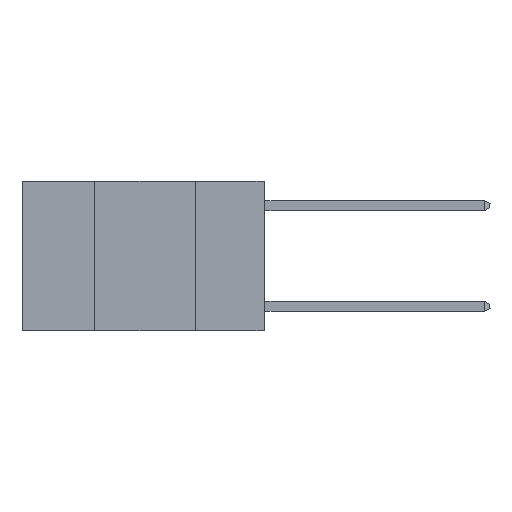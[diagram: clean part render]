
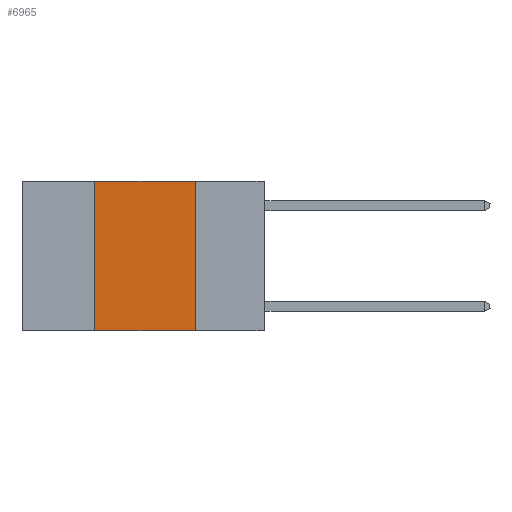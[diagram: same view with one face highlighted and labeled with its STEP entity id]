
A CAD part, left-side view. The second image highlights one B-rep face of the part: STEP entity #6965.
In plain terms, the highlighted planar face has unit normal (-1, 0, 0).
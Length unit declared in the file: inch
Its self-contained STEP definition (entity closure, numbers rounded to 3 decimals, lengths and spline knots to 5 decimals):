
#313 = EDGE_LOOP ( 'NONE', ( #2954, #5446, #2824, #8068 ) ) ;
#497 = CARTESIAN_POINT ( 'NONE',  ( 0., 0.6, 0. ) ) ;
#571 = EDGE_CURVE ( 'NONE', #6247, #1300, #6232, .T. ) ;
#786 = LINE ( 'NONE', #5192, #2354 ) ;
#1005 = CARTESIAN_POINT ( 'NONE',  ( 0., 0.17, -0.37 ) ) ;
#1020 = DIRECTION ( 'NONE',  ( 0., -1., 0. ) ) ;
#1263 = CARTESIAN_POINT ( 'NONE',  ( 0., 0.42, -0.37 ) ) ;
#1300 = VERTEX_POINT ( 'NONE', #2081 ) ;
#1341 = LINE ( 'NONE', #1488, #8252 ) ;
#1369 = VECTOR ( 'NONE', #8205, 39.37008 ) ;
#1441 = DIRECTION ( 'NONE',  ( 0., 0., 1. ) ) ;
#1488 = CARTESIAN_POINT ( 'NONE',  ( 0., 0.42, 0. ) ) ;
#1501 = DIRECTION ( 'NONE',  ( 0., 0., -1. ) ) ;
#2030 = FACE_OUTER_BOUND ( 'NONE', #313, .T. ) ;
#2081 = CARTESIAN_POINT ( 'NONE',  ( 0., 0.17, 0. ) ) ;
#2354 = VECTOR ( 'NONE', #1501, 39.37008 ) ;
#2787 = CARTESIAN_POINT ( 'NONE',  ( 0., 0.42, 0. ) ) ;
#2824 = ORIENTED_EDGE ( 'NONE', *, *, #7184, .F. ) ;
#2954 = ORIENTED_EDGE ( 'NONE', *, *, #6688, .F. ) ;
#3457 = VERTEX_POINT ( 'NONE', #1005 ) ;
#3526 = CARTESIAN_POINT ( 'NONE',  ( 0., 0.6, -0.37 ) ) ;
#4370 = DIRECTION ( 'NONE',  ( 1., 0., 0. ) ) ;
#4730 = VERTEX_POINT ( 'NONE', #1263 ) ;
#5192 = CARTESIAN_POINT ( 'NONE',  ( 0., 0.17, 0. ) ) ;
#5433 = AXIS2_PLACEMENT_3D ( 'NONE', #497, #4370, #5665 ) ;
#5446 = ORIENTED_EDGE ( 'NONE', *, *, #571, .F. ) ;
#5454 = CARTESIAN_POINT ( 'NONE',  ( 0., 0.6, 0. ) ) ;
#5665 = DIRECTION ( 'NONE',  ( 0., 0., -1. ) ) ;
#5813 = PLANE ( 'NONE',  #5433 ) ;
#6232 = LINE ( 'NONE', #5454, #9491 ) ;
#6247 = VERTEX_POINT ( 'NONE', #2787 ) ;
#6688 = EDGE_CURVE ( 'NONE', #1300, #3457, #786, .T. ) ;
#6965 = ADVANCED_FACE ( 'NONE', ( #2030 ), #5813, .F. ) ;
#7173 = EDGE_CURVE ( 'NONE', #4730, #3457, #9038, .T. ) ;
#7184 = EDGE_CURVE ( 'NONE', #4730, #6247, #1341, .T. ) ;
#8068 = ORIENTED_EDGE ( 'NONE', *, *, #7173, .T. ) ;
#8205 = DIRECTION ( 'NONE',  ( 0., -1., 0. ) ) ;
#8252 = VECTOR ( 'NONE', #1441, 39.37008 ) ;
#9038 = LINE ( 'NONE', #3526, #1369 ) ;
#9491 = VECTOR ( 'NONE', #1020, 39.37008 ) ;
